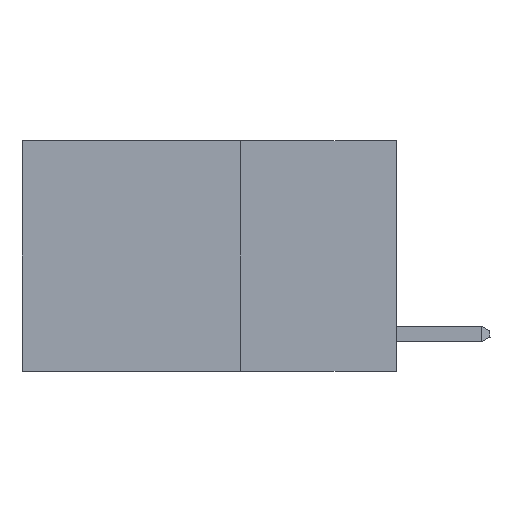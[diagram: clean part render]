
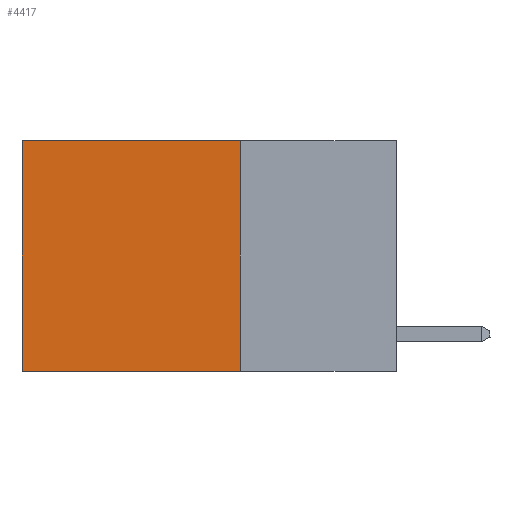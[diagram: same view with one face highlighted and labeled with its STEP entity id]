
A CAD part, left-side view. The second image highlights one B-rep face of the part: STEP entity #4417.
In plain terms, the highlighted planar face has unit normal (-1, 0, 0).
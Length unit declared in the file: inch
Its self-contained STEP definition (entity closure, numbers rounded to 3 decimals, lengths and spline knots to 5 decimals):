
#25 = CARTESIAN_POINT ( 'NONE',  ( 0.2625, 0.25, -0.37 ) ) ;
#51 = VERTEX_POINT ( 'NONE', #2659 ) ;
#53 = DIRECTION ( 'NONE',  ( 0., 0., -1. ) ) ;
#713 = DIRECTION ( 'NONE',  ( 0., 0., -1. ) ) ;
#967 = CARTESIAN_POINT ( 'NONE',  ( 0.2625, 0.25, 0. ) ) ;
#1071 = VERTEX_POINT ( 'NONE', #967 ) ;
#1198 = EDGE_CURVE ( 'NONE', #1071, #2374, #2072, .T. ) ;
#1335 = VERTEX_POINT ( 'NONE', #8546 ) ;
#2072 = LINE ( 'NONE', #4135, #10185 ) ;
#2374 = VERTEX_POINT ( 'NONE', #2720 ) ;
#2659 = CARTESIAN_POINT ( 'NONE',  ( 0.2625, 0.6, 0. ) ) ;
#2720 = CARTESIAN_POINT ( 'NONE',  ( 0.2625, 0.25, -0.37 ) ) ;
#3383 = CARTESIAN_POINT ( 'NONE',  ( 0.2625, 0.25, 0. ) ) ;
#3400 = EDGE_CURVE ( 'NONE', #2374, #1335, #5100, .T. ) ;
#3648 = VECTOR ( 'NONE', #8066, 39.37008 ) ;
#4055 = EDGE_CURVE ( 'NONE', #51, #1335, #9362, .T. ) ;
#4135 = CARTESIAN_POINT ( 'NONE',  ( 0.2625, 0.25, 0. ) ) ;
#4157 = CARTESIAN_POINT ( 'NONE',  ( 0.2625, 0.6, 0. ) ) ;
#4417 = ADVANCED_FACE ( 'NONE', ( #10069 ), #9434, .F. ) ;
#4761 = CARTESIAN_POINT ( 'NONE',  ( 0.2625, 0.25, 0. ) ) ;
#4895 = DIRECTION ( 'NONE',  ( 0., 1., 0. ) ) ;
#5100 = LINE ( 'NONE', #25, #7182 ) ;
#5105 = EDGE_LOOP ( 'NONE', ( #9067, #5149, #7230, #9303 ) ) ;
#5149 = ORIENTED_EDGE ( 'NONE', *, *, #3400, .F. ) ;
#5458 = VECTOR ( 'NONE', #53, 39.37008 ) ;
#5548 = DIRECTION ( 'NONE',  ( 1., 0., 0. ) ) ;
#5743 = LINE ( 'NONE', #3383, #3648 ) ;
#6713 = DIRECTION ( 'NONE',  ( 0., 0., -1. ) ) ;
#7182 = VECTOR ( 'NONE', #4895, 39.37008 ) ;
#7230 = ORIENTED_EDGE ( 'NONE', *, *, #1198, .F. ) ;
#8066 = DIRECTION ( 'NONE',  ( 0., 1., 0. ) ) ;
#8242 = EDGE_CURVE ( 'NONE', #1071, #51, #5743, .T. ) ;
#8546 = CARTESIAN_POINT ( 'NONE',  ( 0.2625, 0.6, -0.37 ) ) ;
#8718 = AXIS2_PLACEMENT_3D ( 'NONE', #4761, #5548, #713 ) ;
#9067 = ORIENTED_EDGE ( 'NONE', *, *, #4055, .T. ) ;
#9303 = ORIENTED_EDGE ( 'NONE', *, *, #8242, .T. ) ;
#9362 = LINE ( 'NONE', #4157, #5458 ) ;
#9434 = PLANE ( 'NONE',  #8718 ) ;
#10069 = FACE_OUTER_BOUND ( 'NONE', #5105, .T. ) ;
#10185 = VECTOR ( 'NONE', #6713, 39.37008 ) ;
